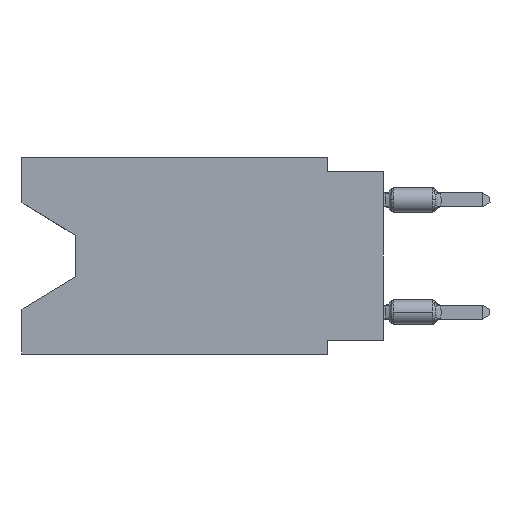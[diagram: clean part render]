
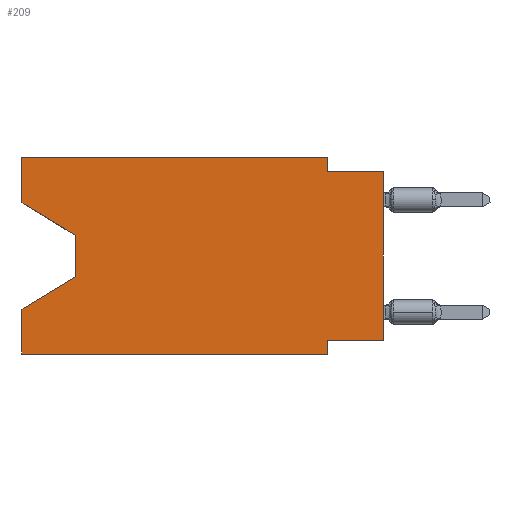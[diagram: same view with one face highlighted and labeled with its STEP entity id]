
A CAD part, left-side view. The second image highlights one B-rep face of the part: STEP entity #209.
In plain terms, the highlighted planar face has unit normal (-1, 0, 0).
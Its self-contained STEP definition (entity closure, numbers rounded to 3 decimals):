
#209 = ADVANCED_FACE ( 'NONE', ( #16318 ), #1585, .F. ) ;
#482 = CARTESIAN_POINT ( 'NONE',  ( 0., 16.383, -2.038 ) ) ;
#1058 = LINE ( 'NONE', #6346, #1521 ) ;
#1105 = CARTESIAN_POINT ( 'NONE',  ( 0., 16.383, -8.89 ) ) ;
#1293 = CARTESIAN_POINT ( 'NONE',  ( 0., 16.383, 0. ) ) ;
#1319 = CARTESIAN_POINT ( 'NONE',  ( 0., 16.383, -6.852 ) ) ;
#1357 = EDGE_CURVE ( 'NONE', #12626, #5036, #13036, .T. ) ;
#1380 = CARTESIAN_POINT ( 'NONE',  ( 0., 16.383, -2.038 ) ) ;
#1521 = VECTOR ( 'NONE', #6508, 1000. ) ;
#1531 = DIRECTION ( 'NONE',  ( 0., 0., -1. ) ) ;
#1585 = PLANE ( 'NONE',  #13974 ) ;
#1901 = CARTESIAN_POINT ( 'NONE',  ( 0., 0., -8.255 ) ) ;
#2186 = VERTEX_POINT ( 'NONE', #16718 ) ;
#2286 = EDGE_CURVE ( 'NONE', #3069, #7848, #6483, .T. ) ;
#3069 = VERTEX_POINT ( 'NONE', #482 ) ;
#3784 = EDGE_CURVE ( 'NONE', #7420, #12175, #5390, .T. ) ;
#3937 = CARTESIAN_POINT ( 'NONE',  ( 0., 16.383, 0. ) ) ;
#3942 = CARTESIAN_POINT ( 'NONE',  ( 0., 0., -0.635 ) ) ;
#4139 = LINE ( 'NONE', #13401, #10142 ) ;
#4257 = DIRECTION ( 'NONE',  ( 0., 0., 1. ) ) ;
#4275 = DIRECTION ( 'NONE',  ( 0., 0., -1. ) ) ;
#4481 = ORIENTED_EDGE ( 'NONE', *, *, #6748, .F. ) ;
#4482 = VERTEX_POINT ( 'NONE', #5093 ) ;
#4706 = EDGE_CURVE ( 'NONE', #12626, #12917, #16405, .T. ) ;
#5036 = VERTEX_POINT ( 'NONE', #6857 ) ;
#5093 = CARTESIAN_POINT ( 'NONE',  ( 0., 2.54, -0.635 ) ) ;
#5247 = ORIENTED_EDGE ( 'NONE', *, *, #16315, .F. ) ;
#5287 = VERTEX_POINT ( 'NONE', #6495 ) ;
#5322 = DIRECTION ( 'NONE',  ( 0., 1., 0. ) ) ;
#5390 = LINE ( 'NONE', #8329, #8480 ) ;
#5417 = LINE ( 'NONE', #5499, #16016 ) ;
#5499 = CARTESIAN_POINT ( 'NONE',  ( 0., 2.54, -8.89 ) ) ;
#6116 = LINE ( 'NONE', #16600, #12613 ) ;
#6248 = CARTESIAN_POINT ( 'NONE',  ( 0., 2.54, 0. ) ) ;
#6346 = CARTESIAN_POINT ( 'NONE',  ( 0., 13.97, -5.385 ) ) ;
#6429 = CARTESIAN_POINT ( 'NONE',  ( 0., 13.97, -3.505 ) ) ;
#6483 = LINE ( 'NONE', #1380, #8131 ) ;
#6495 = CARTESIAN_POINT ( 'NONE',  ( 0., 16.383, 0. ) ) ;
#6508 = DIRECTION ( 'NONE',  ( 0., 0.855, -0.519 ) ) ;
#6717 = EDGE_CURVE ( 'NONE', #2186, #15146, #1058, .T. ) ;
#6748 = EDGE_CURVE ( 'NONE', #3069, #5287, #12054, .T. ) ;
#6783 = CARTESIAN_POINT ( 'NONE',  ( 0., 0., -8.255 ) ) ;
#6857 = CARTESIAN_POINT ( 'NONE',  ( 0., 2.54, -8.255 ) ) ;
#6909 = CARTESIAN_POINT ( 'NONE',  ( 0., 0., -0.635 ) ) ;
#7226 = DIRECTION ( 'NONE',  ( 0., 0., 1. ) ) ;
#7420 = VERTEX_POINT ( 'NONE', #1105 ) ;
#7581 = DIRECTION ( 'NONE',  ( 0., 0., -1. ) ) ;
#7848 = VERTEX_POINT ( 'NONE', #6429 ) ;
#7982 = CARTESIAN_POINT ( 'NONE',  ( 0., 16.383, 0. ) ) ;
#8131 = VECTOR ( 'NONE', #11948, 1000. ) ;
#8329 = CARTESIAN_POINT ( 'NONE',  ( 0., 16.383, -8.89 ) ) ;
#8480 = VECTOR ( 'NONE', #10675, 1000. ) ;
#9005 = VECTOR ( 'NONE', #4257, 1000. ) ;
#9084 = EDGE_CURVE ( 'NONE', #5287, #11245, #15983, .T. ) ;
#9140 = VECTOR ( 'NONE', #14542, 1000. ) ;
#9399 = VECTOR ( 'NONE', #7226, 1000. ) ;
#9855 = EDGE_CURVE ( 'NONE', #7848, #2186, #4139, .T. ) ;
#9917 = ORIENTED_EDGE ( 'NONE', *, *, #16517, .F. ) ;
#10142 = VECTOR ( 'NONE', #1531, 1000. ) ;
#10179 = CARTESIAN_POINT ( 'NONE',  ( 0., 0., 0. ) ) ;
#10212 = EDGE_CURVE ( 'NONE', #11245, #4482, #6116, .T. ) ;
#10292 = ORIENTED_EDGE ( 'NONE', *, *, #10212, .F. ) ;
#10608 = DIRECTION ( 'NONE',  ( 0., -1., 0. ) ) ;
#10675 = DIRECTION ( 'NONE',  ( 0., -1., 0. ) ) ;
#10777 = DIRECTION ( 'NONE',  ( 1., 0., 0. ) ) ;
#10862 = CARTESIAN_POINT ( 'NONE',  ( 0., 16.383, 0. ) ) ;
#10894 = EDGE_LOOP ( 'NONE', ( #14838, #15569, #12516, #17097, #13002, #9917, #11262, #12302, #5247, #10292, #13337, #4481 ) ) ;
#11245 = VERTEX_POINT ( 'NONE', #6248 ) ;
#11262 = ORIENTED_EDGE ( 'NONE', *, *, #1357, .F. ) ;
#11666 = DIRECTION ( 'NONE',  ( 0., -1., 0. ) ) ;
#11786 = VECTOR ( 'NONE', #5322, 1000. ) ;
#11948 = DIRECTION ( 'NONE',  ( 0., -0.855, -0.519 ) ) ;
#12054 = LINE ( 'NONE', #7982, #9005 ) ;
#12070 = CARTESIAN_POINT ( 'NONE',  ( 0., 2.54, -8.89 ) ) ;
#12175 = VERTEX_POINT ( 'NONE', #12070 ) ;
#12302 = ORIENTED_EDGE ( 'NONE', *, *, #4706, .T. ) ;
#12516 = ORIENTED_EDGE ( 'NONE', *, *, #6717, .T. ) ;
#12613 = VECTOR ( 'NONE', #7581, 1000. ) ;
#12626 = VERTEX_POINT ( 'NONE', #1901 ) ;
#12702 = VECTOR ( 'NONE', #11666, 1000. ) ;
#12917 = VERTEX_POINT ( 'NONE', #6909 ) ;
#13002 = ORIENTED_EDGE ( 'NONE', *, *, #3784, .T. ) ;
#13036 = LINE ( 'NONE', #6783, #11786 ) ;
#13337 = ORIENTED_EDGE ( 'NONE', *, *, #9084, .F. ) ;
#13401 = CARTESIAN_POINT ( 'NONE',  ( 0., 13.97, -3.505 ) ) ;
#13667 = VECTOR ( 'NONE', #10608, 1000. ) ;
#13974 = AXIS2_PLACEMENT_3D ( 'NONE', #10862, #10777, #4275 ) ;
#14256 = LINE ( 'NONE', #3942, #12702 ) ;
#14286 = EDGE_CURVE ( 'NONE', #7420, #15146, #14290, .T. ) ;
#14290 = LINE ( 'NONE', #1293, #9140 ) ;
#14542 = DIRECTION ( 'NONE',  ( 0., 0., 1. ) ) ;
#14838 = ORIENTED_EDGE ( 'NONE', *, *, #2286, .T. ) ;
#14942 = DIRECTION ( 'NONE',  ( 0., 0., -1. ) ) ;
#15146 = VERTEX_POINT ( 'NONE', #1319 ) ;
#15569 = ORIENTED_EDGE ( 'NONE', *, *, #9855, .T. ) ;
#15983 = LINE ( 'NONE', #3937, #13667 ) ;
#16016 = VECTOR ( 'NONE', #14942, 1000. ) ;
#16315 = EDGE_CURVE ( 'NONE', #4482, #12917, #14256, .T. ) ;
#16318 = FACE_OUTER_BOUND ( 'NONE', #10894, .T. ) ;
#16405 = LINE ( 'NONE', #10179, #9399 ) ;
#16517 = EDGE_CURVE ( 'NONE', #5036, #12175, #5417, .T. ) ;
#16600 = CARTESIAN_POINT ( 'NONE',  ( 0., 2.54, 0. ) ) ;
#16718 = CARTESIAN_POINT ( 'NONE',  ( 0., 13.97, -5.385 ) ) ;
#17097 = ORIENTED_EDGE ( 'NONE', *, *, #14286, .F. ) ;
